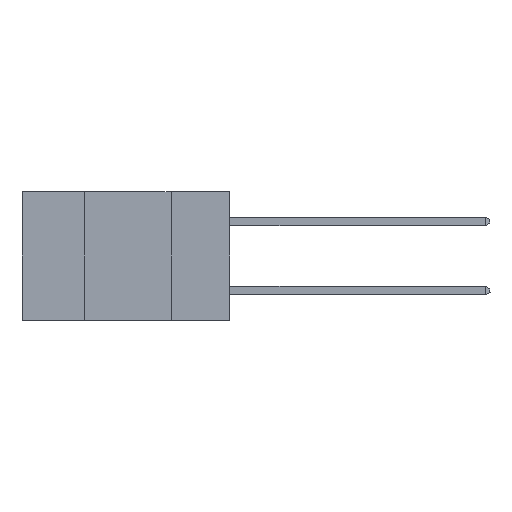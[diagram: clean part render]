
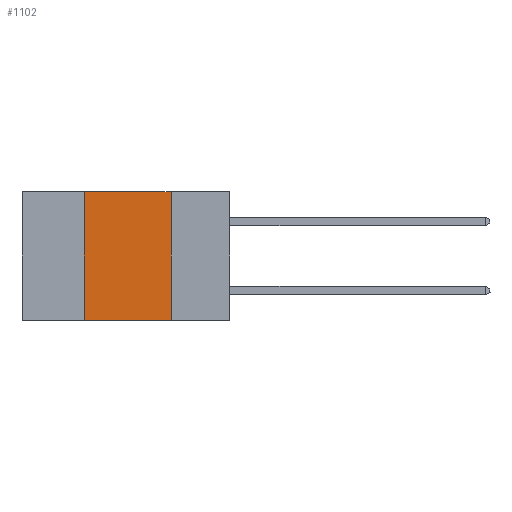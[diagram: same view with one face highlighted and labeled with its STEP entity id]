
A CAD part, left-side view. The second image highlights one B-rep face of the part: STEP entity #1102.
In plain terms, the highlighted planar face has unit normal (-1, 0, 0).
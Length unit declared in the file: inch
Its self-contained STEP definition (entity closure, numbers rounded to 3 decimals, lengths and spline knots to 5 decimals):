
#120 = VERTEX_POINT ( 'NONE', #12575 ) ;
#1035 = VERTEX_POINT ( 'NONE', #9592 ) ;
#1102 = ADVANCED_FACE ( 'NONE', ( #1686 ), #6548, .F. ) ;
#1180 = LINE ( 'NONE', #10346, #5334 ) ;
#1686 = FACE_OUTER_BOUND ( 'NONE', #12455, .T. ) ;
#2284 = CARTESIAN_POINT ( 'NONE',  ( 0., 0.17, 0. ) ) ;
#2314 = DIRECTION ( 'NONE',  ( 0., 0., -1. ) ) ;
#3164 = VERTEX_POINT ( 'NONE', #8817 ) ;
#3434 = DIRECTION ( 'NONE',  ( 0., 0., -1. ) ) ;
#3824 = EDGE_CURVE ( 'NONE', #4683, #3164, #1180, .T. ) ;
#3890 = EDGE_CURVE ( 'NONE', #1035, #120, #7664, .T. ) ;
#4599 = CARTESIAN_POINT ( 'NONE',  ( 0., 0.6, 0. ) ) ;
#4683 = VERTEX_POINT ( 'NONE', #11728 ) ;
#4932 = EDGE_CURVE ( 'NONE', #3164, #1035, #14036, .T. ) ;
#5334 = VECTOR ( 'NONE', #12685, 39.37008 ) ;
#5571 = ORIENTED_EDGE ( 'NONE', *, *, #3824, .F. ) ;
#5594 = ORIENTED_EDGE ( 'NONE', *, *, #14223, .T. ) ;
#5687 = VECTOR ( 'NONE', #14312, 39.37008 ) ;
#5979 = ORIENTED_EDGE ( 'NONE', *, *, #4932, .F. ) ;
#6548 = PLANE ( 'NONE',  #9196 ) ;
#7529 = VECTOR ( 'NONE', #13238, 39.37008 ) ;
#7664 = LINE ( 'NONE', #2284, #12563 ) ;
#8155 = DIRECTION ( 'NONE',  ( 1., 0., 0. ) ) ;
#8817 = CARTESIAN_POINT ( 'NONE',  ( 0., 0.42, 0. ) ) ;
#9196 = AXIS2_PLACEMENT_3D ( 'NONE', #10327, #8155, #2314 ) ;
#9592 = CARTESIAN_POINT ( 'NONE',  ( 0., 0.17, 0. ) ) ;
#10327 = CARTESIAN_POINT ( 'NONE',  ( 0., 0.6, 0. ) ) ;
#10346 = CARTESIAN_POINT ( 'NONE',  ( 0., 0.42, 0. ) ) ;
#10830 = CARTESIAN_POINT ( 'NONE',  ( 0., 0.6, -0.37 ) ) ;
#11490 = LINE ( 'NONE', #10830, #7529 ) ;
#11728 = CARTESIAN_POINT ( 'NONE',  ( 0., 0.42, -0.37 ) ) ;
#12455 = EDGE_LOOP ( 'NONE', ( #12984, #5979, #5571, #5594 ) ) ;
#12563 = VECTOR ( 'NONE', #3434, 39.37008 ) ;
#12575 = CARTESIAN_POINT ( 'NONE',  ( 0., 0.17, -0.37 ) ) ;
#12685 = DIRECTION ( 'NONE',  ( 0., 0., 1. ) ) ;
#12984 = ORIENTED_EDGE ( 'NONE', *, *, #3890, .F. ) ;
#13238 = DIRECTION ( 'NONE',  ( 0., -1., 0. ) ) ;
#14036 = LINE ( 'NONE', #4599, #5687 ) ;
#14223 = EDGE_CURVE ( 'NONE', #4683, #120, #11490, .T. ) ;
#14312 = DIRECTION ( 'NONE',  ( 0., -1., 0. ) ) ;
